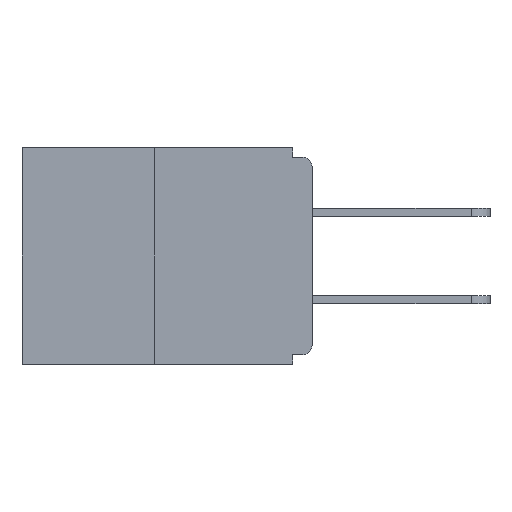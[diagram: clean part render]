
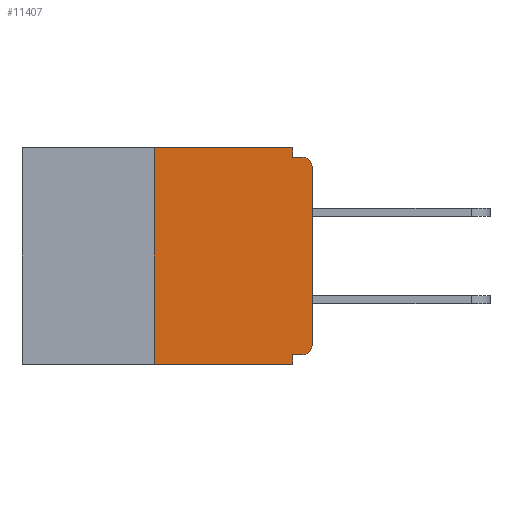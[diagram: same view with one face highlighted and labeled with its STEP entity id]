
A CAD part, left-side view. The second image highlights one B-rep face of the part: STEP entity #11407.
In plain terms, the highlighted planar face has unit normal (-1, 0, 0).
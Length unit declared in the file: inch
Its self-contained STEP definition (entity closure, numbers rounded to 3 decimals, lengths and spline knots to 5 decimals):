
#56 = CARTESIAN_POINT ( 'NONE',  ( 0., 0.031, 0. ) ) ;
#748 = VECTOR ( 'NONE', #11580, 39.37008 ) ;
#806 = ORIENTED_EDGE ( 'NONE', *, *, #1696, .F. ) ;
#874 = AXIS2_PLACEMENT_3D ( 'NONE', #2794, #9230, #6486 ) ;
#1118 = CARTESIAN_POINT ( 'NONE',  ( 0., 0., -0.03 ) ) ;
#1217 = AXIS2_PLACEMENT_3D ( 'NONE', #3205, #9751, #3810 ) ;
#1337 = CARTESIAN_POINT ( 'NONE',  ( 0., 0.015, -0.03 ) ) ;
#1378 = DIRECTION ( 'NONE',  ( 0., 0., -1. ) ) ;
#1397 = VERTEX_POINT ( 'NONE', #9591 ) ;
#1696 = EDGE_CURVE ( 'NONE', #9906, #5753, #5492, .T. ) ;
#1742 = PLANE ( 'NONE',  #874 ) ;
#1769 = FACE_OUTER_BOUND ( 'NONE', #9306, .T. ) ;
#2072 = VECTOR ( 'NONE', #10984, 39.37008 ) ;
#2120 = VECTOR ( 'NONE', #2431, 39.37008 ) ;
#2280 = CARTESIAN_POINT ( 'NONE',  ( 0., 0.25, -0.343 ) ) ;
#2431 = DIRECTION ( 'NONE',  ( 0., -1., 0. ) ) ;
#2438 = DIRECTION ( 'NONE',  ( -1., 0., 0. ) ) ;
#2503 = LINE ( 'NONE', #6761, #3104 ) ;
#2551 = CARTESIAN_POINT ( 'NONE',  ( 0., 0.25, 0. ) ) ;
#2566 = CARTESIAN_POINT ( 'NONE',  ( 0., 0.25, 0. ) ) ;
#2655 = VECTOR ( 'NONE', #9542, 39.37008 ) ;
#2794 = CARTESIAN_POINT ( 'NONE',  ( 0., 0.46, 0. ) ) ;
#3104 = VECTOR ( 'NONE', #7814, 39.37008 ) ;
#3205 = CARTESIAN_POINT ( 'NONE',  ( 0., 0.015, -0.313 ) ) ;
#3372 = EDGE_CURVE ( 'NONE', #11878, #8358, #5442, .T. ) ;
#3512 = DIRECTION ( 'NONE',  ( 0., -1., 0. ) ) ;
#3669 = ORIENTED_EDGE ( 'NONE', *, *, #11150, .T. ) ;
#3758 = EDGE_CURVE ( 'NONE', #10450, #11878, #2503, .T. ) ;
#3810 = DIRECTION ( 'NONE',  ( 0., 0., -1. ) ) ;
#4038 = VERTEX_POINT ( 'NONE', #2551 ) ;
#4201 = VERTEX_POINT ( 'NONE', #7474 ) ;
#4365 = CARTESIAN_POINT ( 'NONE',  ( 0., 0., -0.015 ) ) ;
#4432 = LINE ( 'NONE', #2566, #2072 ) ;
#4511 = CARTESIAN_POINT ( 'NONE',  ( 0., 0.46, 0. ) ) ;
#4715 = DIRECTION ( 'NONE',  ( 0., 0., -1. ) ) ;
#4853 = VECTOR ( 'NONE', #5309, 39.37008 ) ;
#5054 = CARTESIAN_POINT ( 'NONE',  ( 0., 0.46, -0.343 ) ) ;
#5309 = DIRECTION ( 'NONE',  ( 0., 0., -1. ) ) ;
#5388 = VECTOR ( 'NONE', #4715, 39.37008 ) ;
#5442 = LINE ( 'NONE', #7250, #4853 ) ;
#5483 = ORIENTED_EDGE ( 'NONE', *, *, #7506, .F. ) ;
#5492 = LINE ( 'NONE', #4365, #2120 ) ;
#5611 = EDGE_CURVE ( 'NONE', #10450, #4201, #7173, .T. ) ;
#5753 = VERTEX_POINT ( 'NONE', #8282 ) ;
#5920 = ORIENTED_EDGE ( 'NONE', *, *, #3758, .F. ) ;
#6486 = DIRECTION ( 'NONE',  ( 0., 0., -1. ) ) ;
#6509 = ORIENTED_EDGE ( 'NONE', *, *, #10659, .F. ) ;
#6565 = ORIENTED_EDGE ( 'NONE', *, *, #11706, .T. ) ;
#6620 = LINE ( 'NONE', #5054, #748 ) ;
#6761 = CARTESIAN_POINT ( 'NONE',  ( 0., 0., -0.328 ) ) ;
#7173 = CIRCLE ( 'NONE', #1217, 0.015 ) ;
#7250 = CARTESIAN_POINT ( 'NONE',  ( 0., 0.031, -0.343 ) ) ;
#7474 = CARTESIAN_POINT ( 'NONE',  ( 0., 0., -0.313 ) ) ;
#7506 = EDGE_CURVE ( 'NONE', #1397, #9906, #7743, .T. ) ;
#7654 = LINE ( 'NONE', #9503, #2655 ) ;
#7689 = CARTESIAN_POINT ( 'NONE',  ( 0., 0.031, -0.343 ) ) ;
#7743 = LINE ( 'NONE', #56, #5388 ) ;
#7814 = DIRECTION ( 'NONE',  ( 0., 1., 0. ) ) ;
#8044 = EDGE_CURVE ( 'NONE', #4038, #1397, #10770, .T. ) ;
#8282 = CARTESIAN_POINT ( 'NONE',  ( 0., 0.015, -0.015 ) ) ;
#8296 = VECTOR ( 'NONE', #3512, 39.37008 ) ;
#8358 = VERTEX_POINT ( 'NONE', #7689 ) ;
#8558 = VERTEX_POINT ( 'NONE', #2280 ) ;
#8798 = ORIENTED_EDGE ( 'NONE', *, *, #5611, .T. ) ;
#8860 = ORIENTED_EDGE ( 'NONE', *, *, #8044, .F. ) ;
#9230 = DIRECTION ( 'NONE',  ( 1., 0., 0. ) ) ;
#9306 = EDGE_LOOP ( 'NONE', ( #8860, #6509, #6565, #10603, #5920, #8798, #11953, #3669, #806, #5483 ) ) ;
#9462 = CARTESIAN_POINT ( 'NONE',  ( 0., 0.031, -0.015 ) ) ;
#9503 = CARTESIAN_POINT ( 'NONE',  ( 0., 0., 0. ) ) ;
#9542 = DIRECTION ( 'NONE',  ( 0., 0., 1. ) ) ;
#9577 = CARTESIAN_POINT ( 'NONE',  ( 0., 0.015, -0.328 ) ) ;
#9591 = CARTESIAN_POINT ( 'NONE',  ( 0., 0.031, 0. ) ) ;
#9734 = AXIS2_PLACEMENT_3D ( 'NONE', #1337, #2438, #1378 ) ;
#9751 = DIRECTION ( 'NONE',  ( -1., 0., 0. ) ) ;
#9878 = VERTEX_POINT ( 'NONE', #1118 ) ;
#9906 = VERTEX_POINT ( 'NONE', #9462 ) ;
#10091 = CIRCLE ( 'NONE', #9734, 0.015 ) ;
#10450 = VERTEX_POINT ( 'NONE', #9577 ) ;
#10603 = ORIENTED_EDGE ( 'NONE', *, *, #3372, .F. ) ;
#10659 = EDGE_CURVE ( 'NONE', #8558, #4038, #4432, .T. ) ;
#10770 = LINE ( 'NONE', #4511, #8296 ) ;
#10984 = DIRECTION ( 'NONE',  ( 0., 0., 1. ) ) ;
#11150 = EDGE_CURVE ( 'NONE', #9878, #5753, #10091, .T. ) ;
#11407 = ADVANCED_FACE ( 'NONE', ( #1769 ), #1742, .F. ) ;
#11580 = DIRECTION ( 'NONE',  ( 0., -1., 0. ) ) ;
#11644 = EDGE_CURVE ( 'NONE', #4201, #9878, #7654, .T. ) ;
#11662 = CARTESIAN_POINT ( 'NONE',  ( 0., 0.031, -0.328 ) ) ;
#11706 = EDGE_CURVE ( 'NONE', #8558, #8358, #6620, .T. ) ;
#11878 = VERTEX_POINT ( 'NONE', #11662 ) ;
#11953 = ORIENTED_EDGE ( 'NONE', *, *, #11644, .T. ) ;
